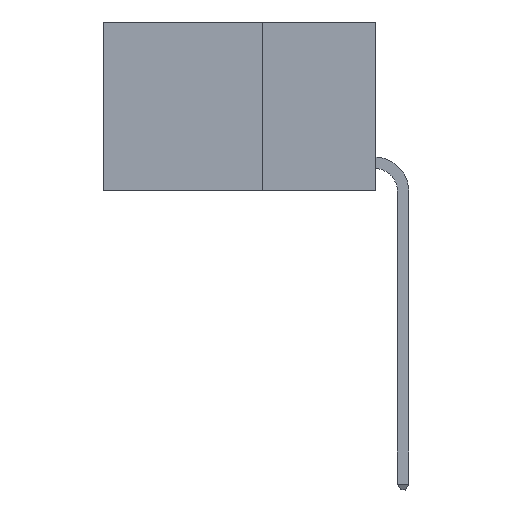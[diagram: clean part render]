
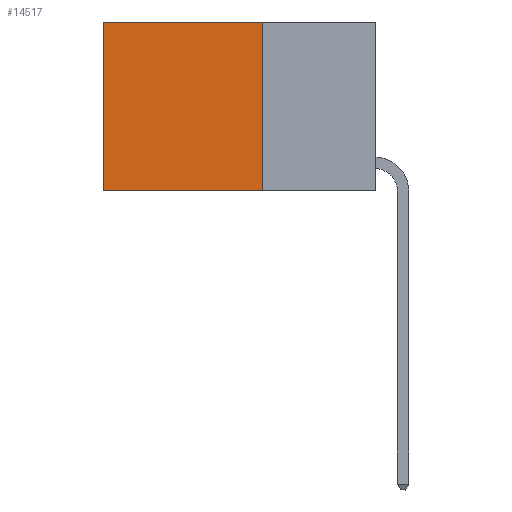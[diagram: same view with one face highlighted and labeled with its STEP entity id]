
A CAD part, left-side view. The second image highlights one B-rep face of the part: STEP entity #14517.
In plain terms, the highlighted planar face has unit normal (-1, 0, 0).
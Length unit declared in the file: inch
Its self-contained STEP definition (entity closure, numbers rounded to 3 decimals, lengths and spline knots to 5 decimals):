
#249 = DIRECTION ( 'NONE',  ( 0., 0., -1. ) ) ;
#558 = VECTOR ( 'NONE', #16096, 39.37008 ) ;
#1341 = VECTOR ( 'NONE', #13791, 39.37008 ) ;
#1406 = EDGE_CURVE ( 'NONE', #13880, #10163, #2926, .T. ) ;
#1994 = CARTESIAN_POINT ( 'NONE',  ( 0.2625, 0.25, 0. ) ) ;
#2671 = CARTESIAN_POINT ( 'NONE',  ( 0.2625, 0.6, 0. ) ) ;
#2926 = LINE ( 'NONE', #7526, #16453 ) ;
#4547 = DIRECTION ( 'NONE',  ( 0., 0., -1. ) ) ;
#4909 = EDGE_LOOP ( 'NONE', ( #15464, #15530, #15574, #15686 ) ) ;
#5046 = LINE ( 'NONE', #19003, #1341 ) ;
#5369 = CARTESIAN_POINT ( 'NONE',  ( 0.2625, 0.6, -0.37 ) ) ;
#5627 = CARTESIAN_POINT ( 'NONE',  ( 0.2625, 0.25, 0. ) ) ;
#5946 = LINE ( 'NONE', #9216, #558 ) ;
#6272 = VERTEX_POINT ( 'NONE', #7161 ) ;
#7161 = CARTESIAN_POINT ( 'NONE',  ( 0.2625, 0.6, 0. ) ) ;
#7526 = CARTESIAN_POINT ( 'NONE',  ( 0.2625, 0.25, 0. ) ) ;
#8015 = EDGE_CURVE ( 'NONE', #6272, #15052, #17075, .T. ) ;
#9216 = CARTESIAN_POINT ( 'NONE',  ( 0.2625, 0.25, 0. ) ) ;
#10163 = VERTEX_POINT ( 'NONE', #20054 ) ;
#10904 = PLANE ( 'NONE',  #16157 ) ;
#10976 = DIRECTION ( 'NONE',  ( 1., 0., 0. ) ) ;
#12491 = VECTOR ( 'NONE', #4547, 39.37008 ) ;
#13791 = DIRECTION ( 'NONE',  ( 0., 1., 0. ) ) ;
#13880 = VERTEX_POINT ( 'NONE', #1994 ) ;
#14517 = ADVANCED_FACE ( 'NONE', ( #15036 ), #10904, .F. ) ;
#15036 = FACE_OUTER_BOUND ( 'NONE', #4909, .T. ) ;
#15052 = VERTEX_POINT ( 'NONE', #5369 ) ;
#15464 = ORIENTED_EDGE ( 'NONE', *, *, #8015, .T. ) ;
#15530 = ORIENTED_EDGE ( 'NONE', *, *, #20630, .F. ) ;
#15574 = ORIENTED_EDGE ( 'NONE', *, *, #1406, .F. ) ;
#15686 = ORIENTED_EDGE ( 'NONE', *, *, #19556, .T. ) ;
#16096 = DIRECTION ( 'NONE',  ( 0., 1., 0. ) ) ;
#16157 = AXIS2_PLACEMENT_3D ( 'NONE', #5627, #10976, #249 ) ;
#16453 = VECTOR ( 'NONE', #19689, 39.37008 ) ;
#17075 = LINE ( 'NONE', #2671, #12491 ) ;
#19003 = CARTESIAN_POINT ( 'NONE',  ( 0.2625, 0.25, -0.37 ) ) ;
#19556 = EDGE_CURVE ( 'NONE', #13880, #6272, #5946, .T. ) ;
#19689 = DIRECTION ( 'NONE',  ( 0., 0., -1. ) ) ;
#20054 = CARTESIAN_POINT ( 'NONE',  ( 0.2625, 0.25, -0.37 ) ) ;
#20630 = EDGE_CURVE ( 'NONE', #10163, #15052, #5046, .T. ) ;
